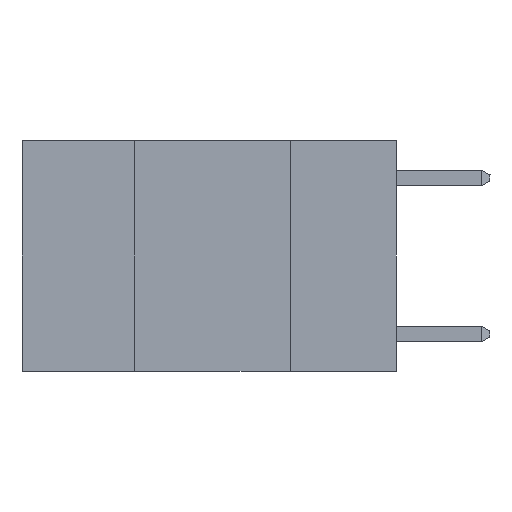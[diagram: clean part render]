
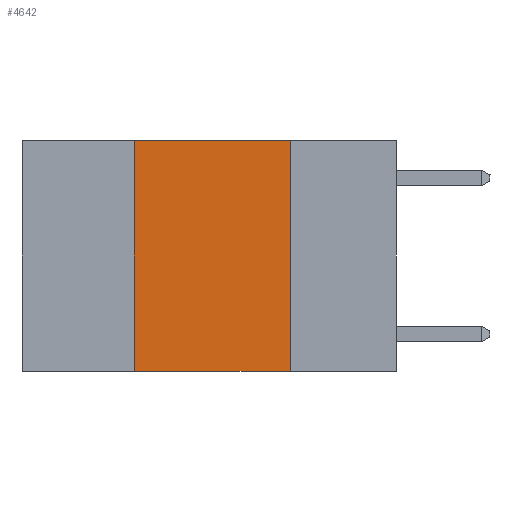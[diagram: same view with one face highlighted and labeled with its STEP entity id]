
A CAD part, left-side view. The second image highlights one B-rep face of the part: STEP entity #4642.
In plain terms, the highlighted planar face has unit normal (-1, 0, 0).
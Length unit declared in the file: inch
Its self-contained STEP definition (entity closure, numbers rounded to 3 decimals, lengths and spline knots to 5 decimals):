
#117 = VERTEX_POINT ( 'NONE', #8215 ) ;
#118 = DIRECTION ( 'NONE',  ( 0., -1., 0. ) ) ;
#596 = EDGE_CURVE ( 'NONE', #117, #7688, #1467, .T. ) ;
#617 = EDGE_LOOP ( 'NONE', ( #8340, #7745, #5217, #1026 ) ) ;
#680 = CARTESIAN_POINT ( 'NONE',  ( 0., 0.6, 0. ) ) ;
#825 = DIRECTION ( 'NONE',  ( 1., 0., 0. ) ) ;
#1008 = CARTESIAN_POINT ( 'NONE',  ( 0., 0.17, 0. ) ) ;
#1026 = ORIENTED_EDGE ( 'NONE', *, *, #1974, .T. ) ;
#1109 = AXIS2_PLACEMENT_3D ( 'NONE', #680, #825, #4473 ) ;
#1421 = CARTESIAN_POINT ( 'NONE',  ( 0., 0.6, -0.37 ) ) ;
#1467 = LINE ( 'NONE', #2987, #6639 ) ;
#1974 = EDGE_CURVE ( 'NONE', #4107, #5758, #2304, .T. ) ;
#2145 = PLANE ( 'NONE',  #1109 ) ;
#2304 = LINE ( 'NONE', #1421, #8156 ) ;
#2987 = CARTESIAN_POINT ( 'NONE',  ( 0., 0.6, 0. ) ) ;
#3473 = CARTESIAN_POINT ( 'NONE',  ( 0., 0.17, -0.37 ) ) ;
#3760 = LINE ( 'NONE', #7640, #5056 ) ;
#4027 = CARTESIAN_POINT ( 'NONE',  ( 0., 0.42, 0. ) ) ;
#4107 = VERTEX_POINT ( 'NONE', #5938 ) ;
#4422 = FACE_OUTER_BOUND ( 'NONE', #617, .T. ) ;
#4473 = DIRECTION ( 'NONE',  ( 0., 0., -1. ) ) ;
#4642 = ADVANCED_FACE ( 'NONE', ( #4422 ), #2145, .F. ) ;
#5056 = VECTOR ( 'NONE', #8244, 39.37008 ) ;
#5217 = ORIENTED_EDGE ( 'NONE', *, *, #8451, .F. ) ;
#5299 = DIRECTION ( 'NONE',  ( 0., -1., 0. ) ) ;
#5534 = VECTOR ( 'NONE', #5578, 39.37008 ) ;
#5578 = DIRECTION ( 'NONE',  ( 0., 0., 1. ) ) ;
#5758 = VERTEX_POINT ( 'NONE', #3473 ) ;
#5938 = CARTESIAN_POINT ( 'NONE',  ( 0., 0.42, -0.37 ) ) ;
#6639 = VECTOR ( 'NONE', #118, 39.37008 ) ;
#7640 = CARTESIAN_POINT ( 'NONE',  ( 0., 0.17, 0. ) ) ;
#7688 = VERTEX_POINT ( 'NONE', #1008 ) ;
#7745 = ORIENTED_EDGE ( 'NONE', *, *, #596, .F. ) ;
#7873 = LINE ( 'NONE', #4027, #5534 ) ;
#8156 = VECTOR ( 'NONE', #5299, 39.37008 ) ;
#8215 = CARTESIAN_POINT ( 'NONE',  ( 0., 0.42, 0. ) ) ;
#8244 = DIRECTION ( 'NONE',  ( 0., 0., -1. ) ) ;
#8269 = EDGE_CURVE ( 'NONE', #7688, #5758, #3760, .T. ) ;
#8340 = ORIENTED_EDGE ( 'NONE', *, *, #8269, .F. ) ;
#8451 = EDGE_CURVE ( 'NONE', #4107, #117, #7873, .T. ) ;
